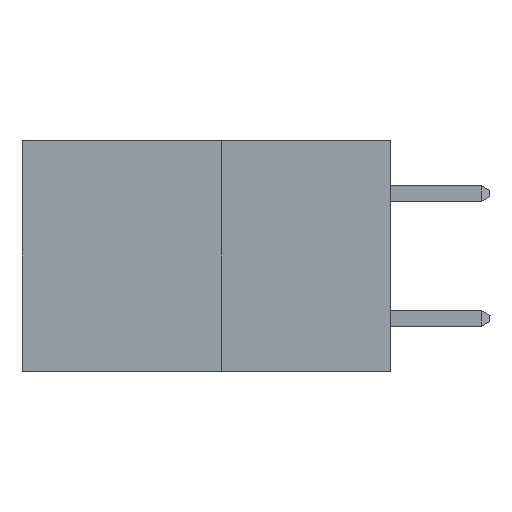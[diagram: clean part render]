
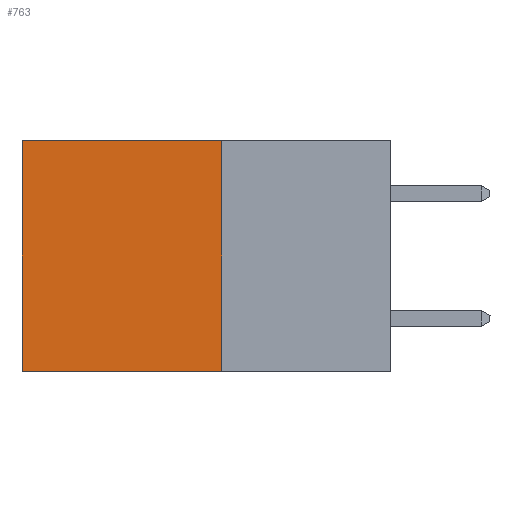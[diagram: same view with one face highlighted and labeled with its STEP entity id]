
A CAD part, left-side view. The second image highlights one B-rep face of the part: STEP entity #763.
In plain terms, the highlighted planar face has unit normal (-1, 0, 0).
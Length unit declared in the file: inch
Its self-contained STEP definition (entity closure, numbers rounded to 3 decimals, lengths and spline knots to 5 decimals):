
#8 = EDGE_CURVE ( 'NONE', #3131, #3298, #5915, .T. ) ;
#763 = ADVANCED_FACE ( 'NONE', ( #5523 ), #8609, .F. ) ;
#915 = VECTOR ( 'NONE', #8186, 39.37008 ) ;
#1142 = ORIENTED_EDGE ( 'NONE', *, *, #8, .F. ) ;
#1186 = LINE ( 'NONE', #8279, #915 ) ;
#1471 = CARTESIAN_POINT ( 'NONE',  ( 0.277, 0.59, 0. ) ) ;
#1636 = VERTEX_POINT ( 'NONE', #6618 ) ;
#1773 = DIRECTION ( 'NONE',  ( 0., 0., -1. ) ) ;
#1776 = EDGE_LOOP ( 'NONE', ( #4979, #1142, #5409, #5881 ) ) ;
#1888 = DIRECTION ( 'NONE',  ( 0., 1., 0. ) ) ;
#2044 = VECTOR ( 'NONE', #3965, 39.37008 ) ;
#2669 = VERTEX_POINT ( 'NONE', #1471 ) ;
#2861 = CARTESIAN_POINT ( 'NONE',  ( 0.277, 0.27, -0.37 ) ) ;
#3131 = VERTEX_POINT ( 'NONE', #5819 ) ;
#3160 = LINE ( 'NONE', #4105, #6791 ) ;
#3196 = CARTESIAN_POINT ( 'NONE',  ( 0.277, 0.27, 0. ) ) ;
#3298 = VERTEX_POINT ( 'NONE', #7703 ) ;
#3965 = DIRECTION ( 'NONE',  ( 0., 1., 0. ) ) ;
#4043 = VECTOR ( 'NONE', #1888, 39.37008 ) ;
#4105 = CARTESIAN_POINT ( 'NONE',  ( 0.277, 0.27, -0.37 ) ) ;
#4476 = EDGE_CURVE ( 'NONE', #2669, #3298, #1186, .T. ) ;
#4479 = CARTESIAN_POINT ( 'NONE',  ( 0.277, 0.27, -0.37 ) ) ;
#4942 = DIRECTION ( 'NONE',  ( 1., 0., 0. ) ) ;
#4979 = ORIENTED_EDGE ( 'NONE', *, *, #4476, .T. ) ;
#5095 = DIRECTION ( 'NONE',  ( 0., 0., -1. ) ) ;
#5409 = ORIENTED_EDGE ( 'NONE', *, *, #9276, .F. ) ;
#5523 = FACE_OUTER_BOUND ( 'NONE', #1776, .T. ) ;
#5819 = CARTESIAN_POINT ( 'NONE',  ( 0.277, 0.27, -0.37 ) ) ;
#5881 = ORIENTED_EDGE ( 'NONE', *, *, #8283, .T. ) ;
#5915 = LINE ( 'NONE', #2861, #4043 ) ;
#5996 = LINE ( 'NONE', #3196, #2044 ) ;
#6433 = AXIS2_PLACEMENT_3D ( 'NONE', #4479, #4942, #5095 ) ;
#6618 = CARTESIAN_POINT ( 'NONE',  ( 0.277, 0.27, 0. ) ) ;
#6791 = VECTOR ( 'NONE', #1773, 39.37008 ) ;
#7703 = CARTESIAN_POINT ( 'NONE',  ( 0.277, 0.59, -0.37 ) ) ;
#8186 = DIRECTION ( 'NONE',  ( 0., 0., -1. ) ) ;
#8279 = CARTESIAN_POINT ( 'NONE',  ( 0.277, 0.59, -0.37 ) ) ;
#8283 = EDGE_CURVE ( 'NONE', #1636, #2669, #5996, .T. ) ;
#8609 = PLANE ( 'NONE',  #6433 ) ;
#9276 = EDGE_CURVE ( 'NONE', #1636, #3131, #3160, .T. ) ;
